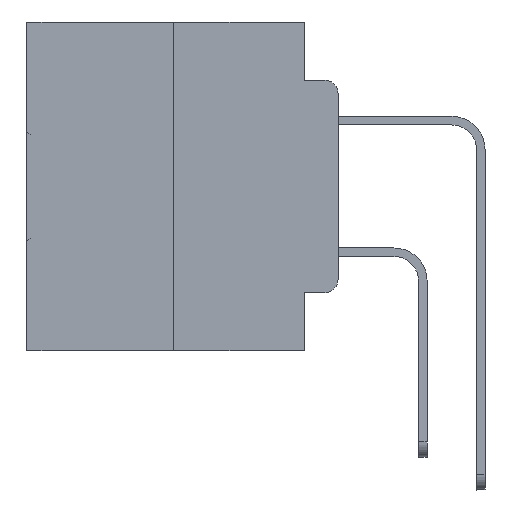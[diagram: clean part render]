
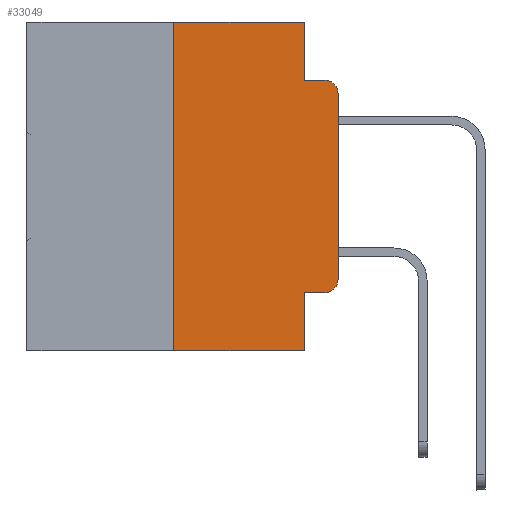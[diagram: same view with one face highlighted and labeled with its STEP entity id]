
A CAD part, left-side view. The second image highlights one B-rep face of the part: STEP entity #33049.
In plain terms, the highlighted planar face has unit normal (-1, 0, 0).
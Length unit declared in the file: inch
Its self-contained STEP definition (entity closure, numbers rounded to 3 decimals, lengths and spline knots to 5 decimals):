
#688 = VECTOR ( 'NONE', #30927, 39.37008 ) ;
#889 = CARTESIAN_POINT ( 'NONE',  ( 0., 0.25, 0. ) ) ;
#1452 = VERTEX_POINT ( 'NONE', #7438 ) ;
#1499 = LINE ( 'NONE', #22730, #28867 ) ;
#1511 = LINE ( 'NONE', #7131, #688 ) ;
#1648 = CARTESIAN_POINT ( 'NONE',  ( 0., 0.051, 0. ) ) ;
#1955 = EDGE_CURVE ( 'NONE', #1452, #3874, #20048, .T. ) ;
#2907 = EDGE_CURVE ( 'NONE', #1452, #9773, #33132, .T. ) ;
#3265 = CARTESIAN_POINT ( 'NONE',  ( 0., 0.051, -0.0885 ) ) ;
#3835 = CARTESIAN_POINT ( 'NONE',  ( 0., 0.25, 0. ) ) ;
#3874 = VERTEX_POINT ( 'NONE', #4028 ) ;
#4028 = CARTESIAN_POINT ( 'NONE',  ( 0., 0.02, -0.4115 ) ) ;
#4410 = VECTOR ( 'NONE', #15749, 39.37008 ) ;
#4733 = DIRECTION ( 'NONE',  ( 0., -1., 0. ) ) ;
#4782 = DIRECTION ( 'NONE',  ( 0., -1., 0. ) ) ;
#4876 = DIRECTION ( 'NONE',  ( 0., -1., 0. ) ) ;
#5094 = VERTEX_POINT ( 'NONE', #889 ) ;
#5713 = CARTESIAN_POINT ( 'NONE',  ( 0., 0.051, -0.4115 ) ) ;
#5944 = EDGE_CURVE ( 'NONE', #22168, #18958, #1511, .T. ) ;
#6067 = ORIENTED_EDGE ( 'NONE', *, *, #13016, .T. ) ;
#6108 = CARTESIAN_POINT ( 'NONE',  ( 0., 0.051, 0. ) ) ;
#6392 = EDGE_CURVE ( 'NONE', #12683, #9773, #14816, .T. ) ;
#6757 = ORIENTED_EDGE ( 'NONE', *, *, #6802, .T. ) ;
#6802 = EDGE_CURVE ( 'NONE', #3874, #14101, #20529, .T. ) ;
#7087 = ORIENTED_EDGE ( 'NONE', *, *, #5944, .F. ) ;
#7131 = CARTESIAN_POINT ( 'NONE',  ( 0., 0.051, -0.0885 ) ) ;
#7432 = CARTESIAN_POINT ( 'NONE',  ( 0., 0., -0.3915 ) ) ;
#7438 = CARTESIAN_POINT ( 'NONE',  ( 0., 0.051, -0.4115 ) ) ;
#7649 = DIRECTION ( 'NONE',  ( -1., 0., 0. ) ) ;
#8653 = DIRECTION ( 'NONE',  ( 0., 0., -1. ) ) ;
#9185 = LINE ( 'NONE', #3835, #29446 ) ;
#9773 = VERTEX_POINT ( 'NONE', #29764 ) ;
#10326 = AXIS2_PLACEMENT_3D ( 'NONE', #15081, #33471, #17757 ) ;
#11741 = EDGE_LOOP ( 'NONE', ( #6067, #13522, #7087, #14974, #22373, #24945, #27419, #20818, #19015, #6757 ) ) ;
#11941 = PLANE ( 'NONE',  #33408 ) ;
#12683 = VERTEX_POINT ( 'NONE', #30040 ) ;
#13016 = EDGE_CURVE ( 'NONE', #14101, #30824, #25554, .T. ) ;
#13522 = ORIENTED_EDGE ( 'NONE', *, *, #14139, .T. ) ;
#14101 = VERTEX_POINT ( 'NONE', #7432 ) ;
#14139 = EDGE_CURVE ( 'NONE', #30824, #18958, #18161, .T. ) ;
#14483 = CARTESIAN_POINT ( 'NONE',  ( 0., 0.02, -0.0885 ) ) ;
#14625 = DIRECTION ( 'NONE',  ( 1., 0., 0. ) ) ;
#14816 = LINE ( 'NONE', #23389, #21832 ) ;
#14974 = ORIENTED_EDGE ( 'NONE', *, *, #21884, .F. ) ;
#15081 = CARTESIAN_POINT ( 'NONE',  ( 0., 0.02, -0.3915 ) ) ;
#15749 = DIRECTION ( 'NONE',  ( 0., 0., 1. ) ) ;
#17183 = DIRECTION ( 'NONE',  ( 0., 0., 1. ) ) ;
#17757 = DIRECTION ( 'NONE',  ( 0., 0., -1. ) ) ;
#18161 = CIRCLE ( 'NONE', #28686, 0.02 ) ;
#18330 = VECTOR ( 'NONE', #8653, 39.37008 ) ;
#18958 = VERTEX_POINT ( 'NONE', #14483 ) ;
#19015 = ORIENTED_EDGE ( 'NONE', *, *, #1955, .T. ) ;
#20048 = LINE ( 'NONE', #5713, #33195 ) ;
#20529 = CIRCLE ( 'NONE', #10326, 0.02 ) ;
#20818 = ORIENTED_EDGE ( 'NONE', *, *, #2907, .F. ) ;
#21624 = FACE_OUTER_BOUND ( 'NONE', #11741, .T. ) ;
#21832 = VECTOR ( 'NONE', #4876, 39.37008 ) ;
#21884 = EDGE_CURVE ( 'NONE', #30679, #22168, #1499, .T. ) ;
#22032 = LINE ( 'NONE', #33724, #28220 ) ;
#22168 = VERTEX_POINT ( 'NONE', #3265 ) ;
#22373 = ORIENTED_EDGE ( 'NONE', *, *, #29442, .F. ) ;
#22730 = CARTESIAN_POINT ( 'NONE',  ( 0., 0.051, 0. ) ) ;
#23389 = CARTESIAN_POINT ( 'NONE',  ( 0., 0.473, -0.5 ) ) ;
#23510 = CARTESIAN_POINT ( 'NONE',  ( 0., 0.02, -0.1085 ) ) ;
#24945 = ORIENTED_EDGE ( 'NONE', *, *, #33020, .F. ) ;
#25554 = LINE ( 'NONE', #31531, #4410 ) ;
#26177 = DIRECTION ( 'NONE',  ( 0., 0., -1. ) ) ;
#27419 = ORIENTED_EDGE ( 'NONE', *, *, #6392, .T. ) ;
#28032 = DIRECTION ( 'NONE',  ( 0., 0., -1. ) ) ;
#28220 = VECTOR ( 'NONE', #4782, 39.37008 ) ;
#28686 = AXIS2_PLACEMENT_3D ( 'NONE', #23510, #7649, #26177 ) ;
#28867 = VECTOR ( 'NONE', #28032, 39.37008 ) ;
#29442 = EDGE_CURVE ( 'NONE', #5094, #30679, #22032, .T. ) ;
#29446 = VECTOR ( 'NONE', #17183, 39.37008 ) ;
#29764 = CARTESIAN_POINT ( 'NONE',  ( 0., 0.051, -0.5 ) ) ;
#30040 = CARTESIAN_POINT ( 'NONE',  ( 0., 0.25, -0.5 ) ) ;
#30389 = CARTESIAN_POINT ( 'NONE',  ( 0., 0.473, 0. ) ) ;
#30679 = VERTEX_POINT ( 'NONE', #1648 ) ;
#30824 = VERTEX_POINT ( 'NONE', #31395 ) ;
#30927 = DIRECTION ( 'NONE',  ( 0., -1., 0. ) ) ;
#31395 = CARTESIAN_POINT ( 'NONE',  ( 0., 0., -0.1085 ) ) ;
#31531 = CARTESIAN_POINT ( 'NONE',  ( 0., 0., 0. ) ) ;
#33020 = EDGE_CURVE ( 'NONE', #12683, #5094, #9185, .T. ) ;
#33032 = DIRECTION ( 'NONE',  ( 0., 0., -1. ) ) ;
#33049 = ADVANCED_FACE ( 'NONE', ( #21624 ), #11941, .F. ) ;
#33132 = LINE ( 'NONE', #6108, #18330 ) ;
#33195 = VECTOR ( 'NONE', #4733, 39.37008 ) ;
#33408 = AXIS2_PLACEMENT_3D ( 'NONE', #30389, #14625, #33032 ) ;
#33471 = DIRECTION ( 'NONE',  ( -1., 0., 0. ) ) ;
#33724 = CARTESIAN_POINT ( 'NONE',  ( 0., 0.473, 0. ) ) ;
